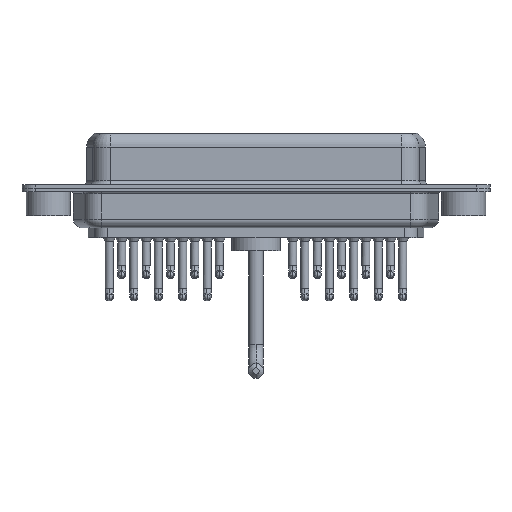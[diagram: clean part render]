
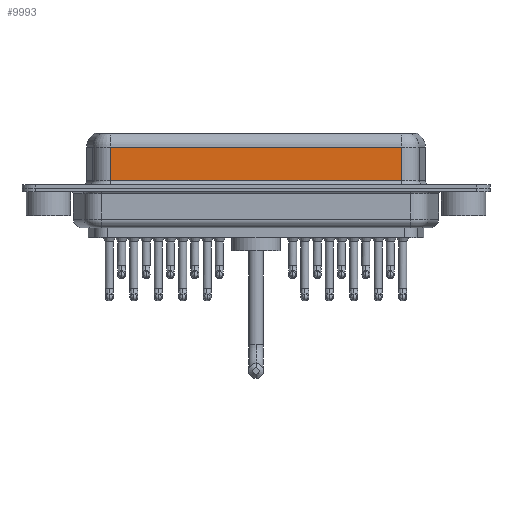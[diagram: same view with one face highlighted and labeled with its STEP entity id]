
A CAD part, front view. The second image highlights one B-rep face of the part: STEP entity #9993.
In plain terms, the highlighted planar face has unit normal (0, -1, 0).
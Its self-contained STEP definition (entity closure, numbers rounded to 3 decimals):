
#926 = CARTESIAN_POINT ( 'NONE',  ( 7.013, -3.95, 6.4 ) ) ;
#965 = DIRECTION ( 'NONE',  ( 1., 0., 0. ) ) ;
#1527 = DIRECTION ( 'NONE',  ( 0., 0., 1. ) ) ;
#2420 = LINE ( 'NONE', #926, #4234 ) ;
#2694 = DIRECTION ( 'NONE',  ( 0., 0., -1. ) ) ;
#3085 = CARTESIAN_POINT ( 'NONE',  ( 40.037, -3.95, 4.65 ) ) ;
#4234 = VECTOR ( 'NONE', #14879, 1000. ) ;
#4847 = ORIENTED_EDGE ( 'NONE', *, *, #21628, .T. ) ;
#5423 = DIRECTION ( 'NONE',  ( 0., 1., 0. ) ) ;
#5922 = EDGE_CURVE ( 'NONE', #7204, #18609, #16577, .T. ) ;
#6594 = ORIENTED_EDGE ( 'NONE', *, *, #11522, .T. ) ;
#6873 = VECTOR ( 'NONE', #11660, 1000. ) ;
#7121 = FACE_OUTER_BOUND ( 'NONE', #19656, .T. ) ;
#7204 = VERTEX_POINT ( 'NONE', #13034 ) ;
#7801 = VERTEX_POINT ( 'NONE', #22384 ) ;
#7877 = VECTOR ( 'NONE', #2694, 1000. ) ;
#7952 = CARTESIAN_POINT ( 'NONE',  ( 40.037, -3.95, 6.4 ) ) ;
#9155 = AXIS2_PLACEMENT_3D ( 'NONE', #18916, #5423, #1527 ) ;
#9537 = CARTESIAN_POINT ( 'NONE',  ( 40.037, -3.95, 0.9 ) ) ;
#9993 = ADVANCED_FACE ( 'NONE', ( #7121 ), #14093, .F. ) ;
#11301 = EDGE_CURVE ( 'NONE', #7204, #17973, #16879, .T. ) ;
#11405 = ORIENTED_EDGE ( 'NONE', *, *, #11301, .F. ) ;
#11522 = EDGE_CURVE ( 'NONE', #18609, #7801, #2420, .T. ) ;
#11660 = DIRECTION ( 'NONE',  ( -1., 0., 0. ) ) ;
#13034 = CARTESIAN_POINT ( 'NONE',  ( 40.037, -3.95, 4.65 ) ) ;
#13461 = ORIENTED_EDGE ( 'NONE', *, *, #5922, .T. ) ;
#14093 = PLANE ( 'NONE',  #9155 ) ;
#14879 = DIRECTION ( 'NONE',  ( 0., 0., -1. ) ) ;
#14921 = VECTOR ( 'NONE', #965, 1000. ) ;
#16115 = CARTESIAN_POINT ( 'NONE',  ( 40.037, -3.95, 0.9 ) ) ;
#16577 = LINE ( 'NONE', #3085, #6873 ) ;
#16879 = LINE ( 'NONE', #7952, #7877 ) ;
#17973 = VERTEX_POINT ( 'NONE', #16115 ) ;
#18234 = LINE ( 'NONE', #9537, #14921 ) ;
#18483 = CARTESIAN_POINT ( 'NONE',  ( 7.013, -3.95, 4.65 ) ) ;
#18609 = VERTEX_POINT ( 'NONE', #18483 ) ;
#18916 = CARTESIAN_POINT ( 'NONE',  ( 40.037, -3.95, 6.4 ) ) ;
#19656 = EDGE_LOOP ( 'NONE', ( #11405, #13461, #6594, #4847 ) ) ;
#21628 = EDGE_CURVE ( 'NONE', #7801, #17973, #18234, .T. ) ;
#22384 = CARTESIAN_POINT ( 'NONE',  ( 7.013, -3.95, 0.9 ) ) ;
